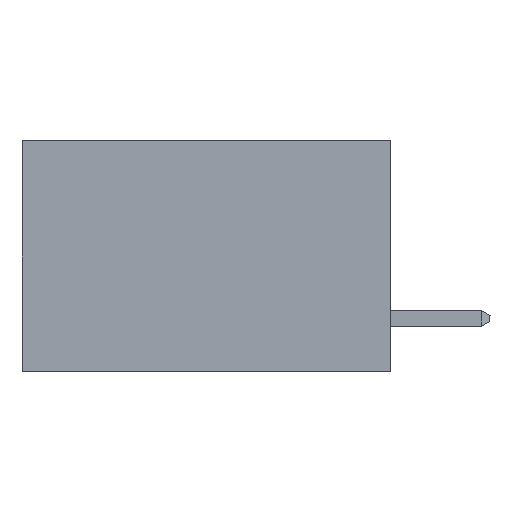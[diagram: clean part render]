
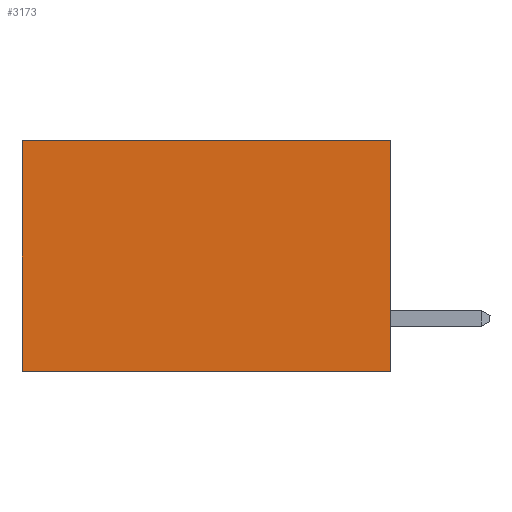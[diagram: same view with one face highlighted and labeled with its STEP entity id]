
A CAD part, left-side view. The second image highlights one B-rep face of the part: STEP entity #3173.
In plain terms, the highlighted planar face has unit normal (-1, 0, 0).
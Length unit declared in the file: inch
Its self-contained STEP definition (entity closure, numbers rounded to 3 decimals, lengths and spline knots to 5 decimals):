
#296 = FACE_OUTER_BOUND ( 'NONE', #6407, .T. ) ;
#528 = EDGE_CURVE ( 'NONE', #5839, #3456, #8642, .T. ) ;
#558 = EDGE_CURVE ( 'NONE', #6242, #5839, #1899, .T. ) ;
#584 = CARTESIAN_POINT ( 'NONE',  ( 0.277, 0.59, -0.37 ) ) ;
#688 = DIRECTION ( 'NONE',  ( 0., 0., -1. ) ) ;
#1536 = CARTESIAN_POINT ( 'NONE',  ( 0.277, 0., -0.37 ) ) ;
#1899 = LINE ( 'NONE', #1536, #9648 ) ;
#1961 = VECTOR ( 'NONE', #6442, 39.37008 ) ;
#2007 = CARTESIAN_POINT ( 'NONE',  ( 0.277, 0., -0.37 ) ) ;
#2416 = VECTOR ( 'NONE', #4450, 39.37008 ) ;
#2995 = CARTESIAN_POINT ( 'NONE',  ( 0.277, 0., -0.37 ) ) ;
#3173 = ADVANCED_FACE ( 'NONE', ( #296 ), #5854, .F. ) ;
#3456 = VERTEX_POINT ( 'NONE', #584 ) ;
#3730 = AXIS2_PLACEMENT_3D ( 'NONE', #2007, #4988, #4976 ) ;
#4450 = DIRECTION ( 'NONE',  ( 0., 1., 0. ) ) ;
#4976 = DIRECTION ( 'NONE',  ( 0., 0., -1. ) ) ;
#4988 = DIRECTION ( 'NONE',  ( 1., 0., 0. ) ) ;
#5152 = EDGE_CURVE ( 'NONE', #6242, #7735, #8483, .T. ) ;
#5696 = CARTESIAN_POINT ( 'NONE',  ( 0.277, 0.59, 0. ) ) ;
#5839 = VERTEX_POINT ( 'NONE', #2995 ) ;
#5854 = PLANE ( 'NONE',  #3730 ) ;
#5917 = EDGE_CURVE ( 'NONE', #7735, #3456, #8463, .T. ) ;
#6163 = DIRECTION ( 'NONE',  ( 0., 0., -1. ) ) ;
#6242 = VERTEX_POINT ( 'NONE', #8048 ) ;
#6407 = EDGE_LOOP ( 'NONE', ( #6790, #6859, #6761, #7481 ) ) ;
#6442 = DIRECTION ( 'NONE',  ( 0., 1., 0. ) ) ;
#6497 = CARTESIAN_POINT ( 'NONE',  ( 0.277, 0., -0.37 ) ) ;
#6711 = CARTESIAN_POINT ( 'NONE',  ( 0.277, 0., 0. ) ) ;
#6761 = ORIENTED_EDGE ( 'NONE', *, *, #558, .F. ) ;
#6790 = ORIENTED_EDGE ( 'NONE', *, *, #5917, .T. ) ;
#6859 = ORIENTED_EDGE ( 'NONE', *, *, #528, .F. ) ;
#7481 = ORIENTED_EDGE ( 'NONE', *, *, #5152, .T. ) ;
#7735 = VERTEX_POINT ( 'NONE', #5696 ) ;
#8048 = CARTESIAN_POINT ( 'NONE',  ( 0.277, 0., 0. ) ) ;
#8463 = LINE ( 'NONE', #9779, #9840 ) ;
#8483 = LINE ( 'NONE', #6711, #1961 ) ;
#8642 = LINE ( 'NONE', #6497, #2416 ) ;
#9648 = VECTOR ( 'NONE', #6163, 39.37008 ) ;
#9779 = CARTESIAN_POINT ( 'NONE',  ( 0.277, 0.59, -0.37 ) ) ;
#9840 = VECTOR ( 'NONE', #688, 39.37008 ) ;
